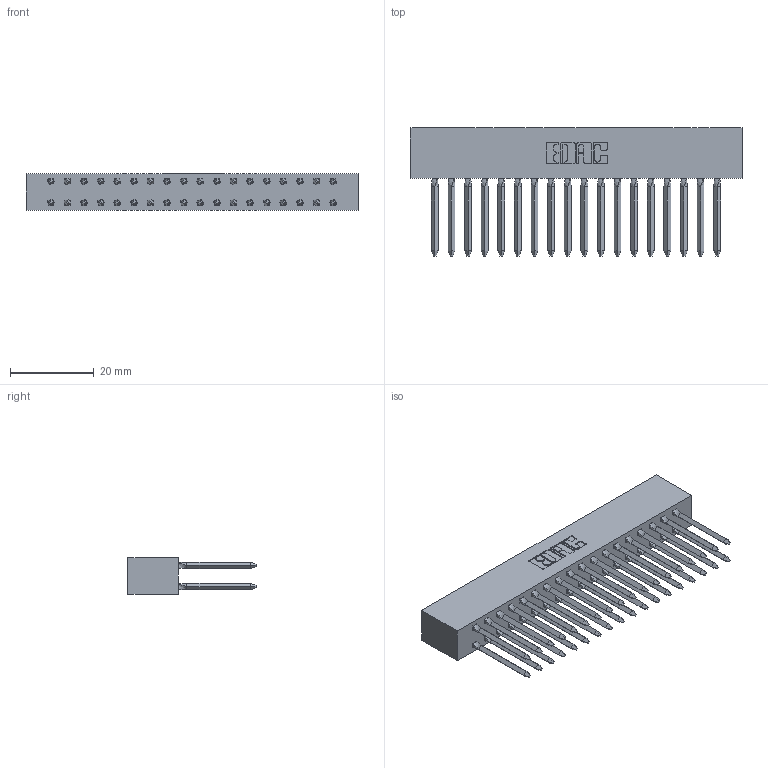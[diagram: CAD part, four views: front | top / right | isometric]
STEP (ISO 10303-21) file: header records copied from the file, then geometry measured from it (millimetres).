
FILE_DESCRIPTION (( 'STEP AP203' ), '1' );
FILE_NAME ('338-036-541-201.STEP', '2020-03-24T18:24:27', ( '' ), ( '' ), 'SwSTEP 2.0', 'SolidWorks 2016', '' );
FILE_SCHEMA (( 'CONFIG_CONTROL_DESIGN' ));
Length unit declared in the file: inch
Products named in the file (3): 338-210-001_338-210-018-001; 338-290-001_541; 338-036-541-201
Assembly tree (37 placements, depth 2):
  338-036-541-201
    338-210-001_338-210-018-001
    338-290-001_541  x36
Bounding box: 79.2 x 30.56 x 8.71 mm (x, y, z)
Volume: 6432.7 mm3; surface area: 12208.1 mm2
Topology: 37 solids, 37 shells, 2498 faces, 6707 edges, 4254 vertices
Faces by surface type: plane 1738, cylinder 616, bspline 144
Entity records: 37350 total; most frequent: CARTESIAN_POINT 7456, ORIENTED_EDGE 6204, DIRECTION 5809, EDGE_CURVE 3102, LINE 2291, VECTOR 2291, VERTEX_POINT 2014, AXIS2_PLACEMENT_3D 1759
